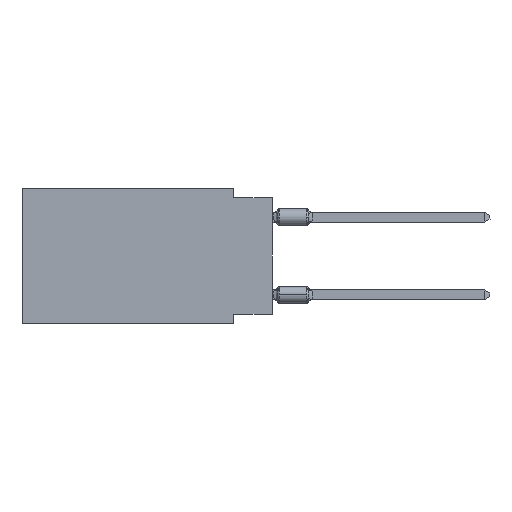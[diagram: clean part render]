
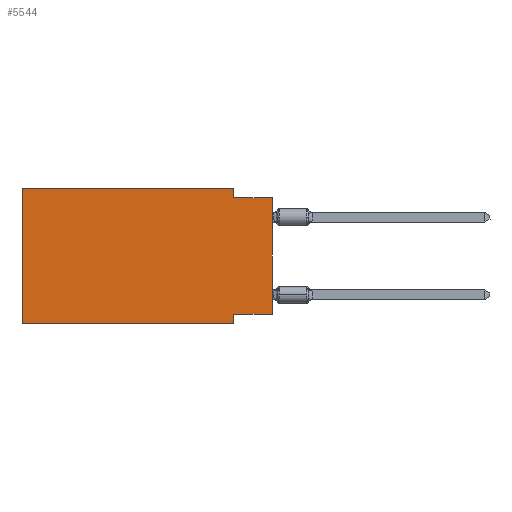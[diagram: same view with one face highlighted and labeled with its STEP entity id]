
A CAD part, left-side view. The second image highlights one B-rep face of the part: STEP entity #5544.
In plain terms, the highlighted planar face has unit normal (-1, 0, 0).
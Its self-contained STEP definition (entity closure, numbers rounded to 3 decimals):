
#216 = VERTEX_POINT ( 'NONE', #6136 ) ;
#246 = VECTOR ( 'NONE', #28995, 1000. ) ;
#1261 = CARTESIAN_POINT ( 'NONE',  ( 0., 2.54, -8.89 ) ) ;
#1277 = DIRECTION ( 'NONE',  ( 0., 0., 1. ) ) ;
#1372 = ORIENTED_EDGE ( 'NONE', *, *, #23637, .F. ) ;
#1504 = LINE ( 'NONE', #3963, #14506 ) ;
#3669 = CARTESIAN_POINT ( 'NONE',  ( 0., 0., -0.635 ) ) ;
#3933 = CARTESIAN_POINT ( 'NONE',  ( 0., 16.383, 0. ) ) ;
#3963 = CARTESIAN_POINT ( 'NONE',  ( 0., 2.54, 0. ) ) ;
#4149 = LINE ( 'NONE', #11688, #11065 ) ;
#4241 = EDGE_LOOP ( 'NONE', ( #7933, #23278, #1372, #27641, #18421, #12700, #15459, #24283 ) ) ;
#4491 = VERTEX_POINT ( 'NONE', #12878 ) ;
#5080 = LINE ( 'NONE', #18811, #17101 ) ;
#5231 = DIRECTION ( 'NONE',  ( 0., 0., -1. ) ) ;
#5544 = ADVANCED_FACE ( 'NONE', ( #14643 ), #25770, .F. ) ;
#5675 = LINE ( 'NONE', #3669, #246 ) ;
#6136 = CARTESIAN_POINT ( 'NONE',  ( 0., 2.54, -0.635 ) ) ;
#6388 = LINE ( 'NONE', #3933, #30263 ) ;
#7933 = ORIENTED_EDGE ( 'NONE', *, *, #9218, .T. ) ;
#8040 = CARTESIAN_POINT ( 'NONE',  ( 0., 2.54, 0. ) ) ;
#8154 = EDGE_CURVE ( 'NONE', #18061, #24471, #18954, .T. ) ;
#9218 = EDGE_CURVE ( 'NONE', #15798, #22716, #17625, .T. ) ;
#9390 = DIRECTION ( 'NONE',  ( 0., 1., 0. ) ) ;
#10743 = CARTESIAN_POINT ( 'NONE',  ( 0., 0., -8.255 ) ) ;
#10997 = EDGE_CURVE ( 'NONE', #12016, #28175, #6388, .T. ) ;
#11065 = VECTOR ( 'NONE', #9390, 1000. ) ;
#11688 = CARTESIAN_POINT ( 'NONE',  ( 0., 0., -8.255 ) ) ;
#12016 = VERTEX_POINT ( 'NONE', #28957 ) ;
#12700 = ORIENTED_EDGE ( 'NONE', *, *, #8154, .T. ) ;
#12878 = CARTESIAN_POINT ( 'NONE',  ( 0., 2.54, -8.255 ) ) ;
#14506 = VECTOR ( 'NONE', #27112, 1000. ) ;
#14643 = FACE_OUTER_BOUND ( 'NONE', #4241, .T. ) ;
#14888 = CARTESIAN_POINT ( 'NONE',  ( 0., 0., -0.635 ) ) ;
#15459 = ORIENTED_EDGE ( 'NONE', *, *, #23232, .F. ) ;
#15798 = VERTEX_POINT ( 'NONE', #10743 ) ;
#16658 = CARTESIAN_POINT ( 'NONE',  ( 0., 16.383, -8.89 ) ) ;
#17101 = VECTOR ( 'NONE', #26078, 1000. ) ;
#17161 = CARTESIAN_POINT ( 'NONE',  ( 0., 2.54, -8.89 ) ) ;
#17625 = LINE ( 'NONE', #27053, #29155 ) ;
#17951 = DIRECTION ( 'NONE',  ( 0., -1., 0. ) ) ;
#18061 = VERTEX_POINT ( 'NONE', #16658 ) ;
#18421 = ORIENTED_EDGE ( 'NONE', *, *, #26634, .F. ) ;
#18654 = CARTESIAN_POINT ( 'NONE',  ( 0., 16.383, 0. ) ) ;
#18811 = CARTESIAN_POINT ( 'NONE',  ( 0., 16.383, 0. ) ) ;
#18954 = LINE ( 'NONE', #28078, #26595 ) ;
#19006 = EDGE_CURVE ( 'NONE', #216, #22716, #5675, .T. ) ;
#20969 = DIRECTION ( 'NONE',  ( 0., -1., 0. ) ) ;
#22716 = VERTEX_POINT ( 'NONE', #14888 ) ;
#22801 = AXIS2_PLACEMENT_3D ( 'NONE', #18654, #23448, #5231 ) ;
#23232 = EDGE_CURVE ( 'NONE', #4491, #24471, #26423, .T. ) ;
#23278 = ORIENTED_EDGE ( 'NONE', *, *, #19006, .F. ) ;
#23448 = DIRECTION ( 'NONE',  ( 1., 0., 0. ) ) ;
#23637 = EDGE_CURVE ( 'NONE', #28175, #216, #1504, .T. ) ;
#24126 = DIRECTION ( 'NONE',  ( 0., 0., -1. ) ) ;
#24283 = ORIENTED_EDGE ( 'NONE', *, *, #25140, .F. ) ;
#24471 = VERTEX_POINT ( 'NONE', #1261 ) ;
#25140 = EDGE_CURVE ( 'NONE', #15798, #4491, #4149, .T. ) ;
#25770 = PLANE ( 'NONE',  #22801 ) ;
#26078 = DIRECTION ( 'NONE',  ( 0., 0., 1. ) ) ;
#26185 = VECTOR ( 'NONE', #24126, 1000. ) ;
#26423 = LINE ( 'NONE', #17161, #26185 ) ;
#26595 = VECTOR ( 'NONE', #20969, 1000. ) ;
#26634 = EDGE_CURVE ( 'NONE', #18061, #12016, #5080, .T. ) ;
#27053 = CARTESIAN_POINT ( 'NONE',  ( 0., 0., 0. ) ) ;
#27112 = DIRECTION ( 'NONE',  ( 0., 0., -1. ) ) ;
#27641 = ORIENTED_EDGE ( 'NONE', *, *, #10997, .F. ) ;
#28078 = CARTESIAN_POINT ( 'NONE',  ( 0., 16.383, -8.89 ) ) ;
#28175 = VERTEX_POINT ( 'NONE', #8040 ) ;
#28957 = CARTESIAN_POINT ( 'NONE',  ( 0., 16.383, 0. ) ) ;
#28995 = DIRECTION ( 'NONE',  ( 0., -1., 0. ) ) ;
#29155 = VECTOR ( 'NONE', #1277, 1000. ) ;
#30263 = VECTOR ( 'NONE', #17951, 1000. ) ;
